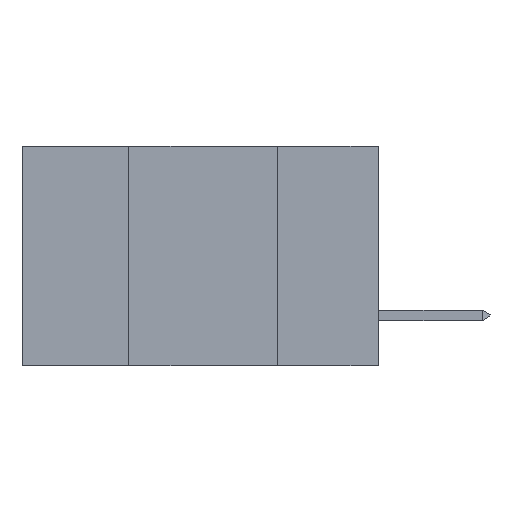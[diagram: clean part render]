
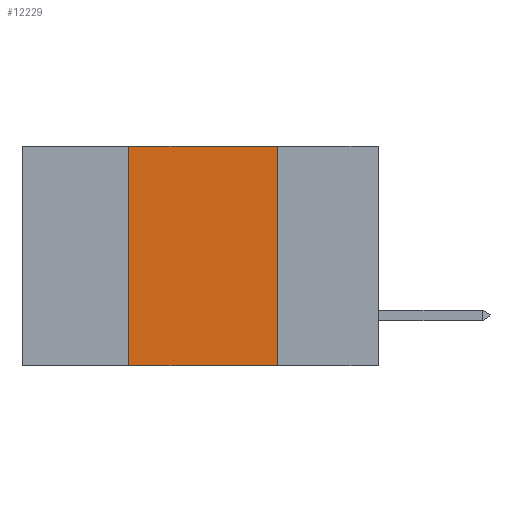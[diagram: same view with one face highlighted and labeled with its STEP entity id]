
A CAD part, left-side view. The second image highlights one B-rep face of the part: STEP entity #12229.
In plain terms, the highlighted planar face has unit normal (-1, 0, 0).
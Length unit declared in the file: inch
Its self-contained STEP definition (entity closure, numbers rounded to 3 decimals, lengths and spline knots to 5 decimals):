
#108 = VERTEX_POINT ( 'NONE', #6080 ) ;
#910 = EDGE_CURVE ( 'NONE', #9489, #11715, #3717, .T. ) ;
#1023 = VERTEX_POINT ( 'NONE', #12489 ) ;
#1150 = DIRECTION ( 'NONE',  ( 0., 0., 1. ) ) ;
#1328 = VECTOR ( 'NONE', #4171, 39.37008 ) ;
#1877 = LINE ( 'NONE', #3254, #11570 ) ;
#2502 = ORIENTED_EDGE ( 'NONE', *, *, #8494, .F. ) ;
#2563 = VECTOR ( 'NONE', #11933, 39.37008 ) ;
#2998 = CARTESIAN_POINT ( 'NONE',  ( 0., 0.6, -0.37 ) ) ;
#3254 = CARTESIAN_POINT ( 'NONE',  ( 0., 0.42, -0.37 ) ) ;
#3384 = ORIENTED_EDGE ( 'NONE', *, *, #910, .F. ) ;
#3514 = FACE_OUTER_BOUND ( 'NONE', #12653, .T. ) ;
#3587 = PLANE ( 'NONE',  #6069 ) ;
#3717 = LINE ( 'NONE', #8066, #5878 ) ;
#4171 = DIRECTION ( 'NONE',  ( 0., 0., -1. ) ) ;
#4270 = CARTESIAN_POINT ( 'NONE',  ( 0., 0.17, 0. ) ) ;
#5623 = ORIENTED_EDGE ( 'NONE', *, *, #6266, .T. ) ;
#5878 = VECTOR ( 'NONE', #9249, 39.37008 ) ;
#5920 = CARTESIAN_POINT ( 'NONE',  ( 0., 0.6, 0. ) ) ;
#6069 = AXIS2_PLACEMENT_3D ( 'NONE', #5920, #9277, #6940 ) ;
#6080 = CARTESIAN_POINT ( 'NONE',  ( 0., 0.42, -0.37 ) ) ;
#6266 = EDGE_CURVE ( 'NONE', #108, #1023, #10919, .T. ) ;
#6940 = DIRECTION ( 'NONE',  ( 0., 0., -1. ) ) ;
#7477 = ORIENTED_EDGE ( 'NONE', *, *, #11109, .F. ) ;
#8066 = CARTESIAN_POINT ( 'NONE',  ( 0., 0.6, 0. ) ) ;
#8494 = EDGE_CURVE ( 'NONE', #11715, #1023, #11789, .T. ) ;
#9249 = DIRECTION ( 'NONE',  ( 0., -1., 0. ) ) ;
#9277 = DIRECTION ( 'NONE',  ( 1., 0., 0. ) ) ;
#9489 = VERTEX_POINT ( 'NONE', #10812 ) ;
#10812 = CARTESIAN_POINT ( 'NONE',  ( 0., 0.42, 0. ) ) ;
#10919 = LINE ( 'NONE', #2998, #2563 ) ;
#11109 = EDGE_CURVE ( 'NONE', #108, #9489, #1877, .T. ) ;
#11570 = VECTOR ( 'NONE', #1150, 39.37008 ) ;
#11715 = VERTEX_POINT ( 'NONE', #4270 ) ;
#11789 = LINE ( 'NONE', #14137, #1328 ) ;
#11933 = DIRECTION ( 'NONE',  ( 0., -1., 0. ) ) ;
#12229 = ADVANCED_FACE ( 'NONE', ( #3514 ), #3587, .F. ) ;
#12489 = CARTESIAN_POINT ( 'NONE',  ( 0., 0.17, -0.37 ) ) ;
#12653 = EDGE_LOOP ( 'NONE', ( #2502, #3384, #7477, #5623 ) ) ;
#14137 = CARTESIAN_POINT ( 'NONE',  ( 0., 0.17, -0.37 ) ) ;
